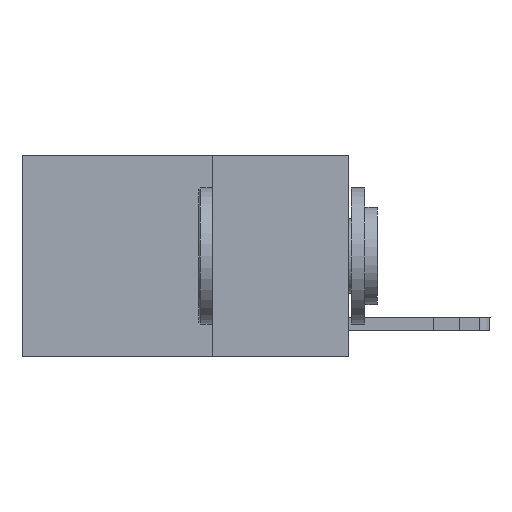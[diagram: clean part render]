
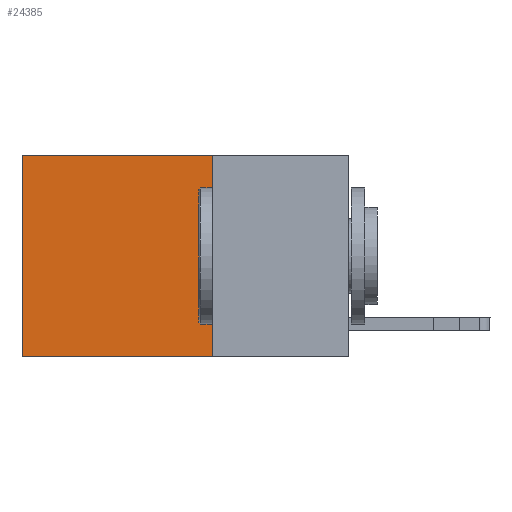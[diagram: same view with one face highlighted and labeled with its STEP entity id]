
A CAD part, left-side view. The second image highlights one B-rep face of the part: STEP entity #24385.
In plain terms, the highlighted planar face has unit normal (-1, 0, 0).
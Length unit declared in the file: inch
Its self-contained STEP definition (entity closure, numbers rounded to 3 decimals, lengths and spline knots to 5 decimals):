
#61 = ORIENTED_EDGE ( 'NONE', *, *, #6524, .T. ) ;
#333 = FACE_OUTER_BOUND ( 'NONE', #22624, .T. ) ;
#690 = EDGE_CURVE ( 'NONE', #24921, #1788, #8399, .T. ) ;
#1788 = VERTEX_POINT ( 'NONE', #17056 ) ;
#2636 = AXIS2_PLACEMENT_3D ( 'NONE', #22788, #10754, #24812 ) ;
#2670 = EDGE_CURVE ( 'NONE', #4900, #24490, #13445, .T. ) ;
#2940 = CARTESIAN_POINT ( 'NONE',  ( 0.2625, 0.6, 0. ) ) ;
#4840 = DIRECTION ( 'NONE',  ( 0., 0., -1. ) ) ;
#4900 = VERTEX_POINT ( 'NONE', #12965 ) ;
#5630 = CARTESIAN_POINT ( 'NONE',  ( 0.2625, 0.25, 0. ) ) ;
#6524 = EDGE_CURVE ( 'NONE', #24490, #1788, #13587, .T. ) ;
#7701 = DIRECTION ( 'NONE',  ( 0., 1., 0. ) ) ;
#7857 = CARTESIAN_POINT ( 'NONE',  ( 0.2625, 0.25, 0. ) ) ;
#8399 = LINE ( 'NONE', #25660, #13099 ) ;
#10754 = DIRECTION ( 'NONE',  ( 1., 0., 0. ) ) ;
#11205 = VECTOR ( 'NONE', #15688, 39.37008 ) ;
#12495 = EDGE_CURVE ( 'NONE', #4900, #24921, #21913, .T. ) ;
#12965 = CARTESIAN_POINT ( 'NONE',  ( 0.2625, 0.25, 0. ) ) ;
#13099 = VECTOR ( 'NONE', #25542, 39.37008 ) ;
#13445 = LINE ( 'NONE', #7857, #18806 ) ;
#13587 = LINE ( 'NONE', #16914, #24276 ) ;
#14439 = CARTESIAN_POINT ( 'NONE',  ( 0.2625, 0.25, -0.37 ) ) ;
#15688 = DIRECTION ( 'NONE',  ( 0., 0., -1. ) ) ;
#16728 = PLANE ( 'NONE',  #2636 ) ;
#16914 = CARTESIAN_POINT ( 'NONE',  ( 0.2625, 0.6, 0. ) ) ;
#17056 = CARTESIAN_POINT ( 'NONE',  ( 0.2625, 0.6, -0.37 ) ) ;
#18497 = ORIENTED_EDGE ( 'NONE', *, *, #2670, .T. ) ;
#18806 = VECTOR ( 'NONE', #7701, 39.37008 ) ;
#20195 = ORIENTED_EDGE ( 'NONE', *, *, #12495, .F. ) ;
#21028 = ORIENTED_EDGE ( 'NONE', *, *, #690, .F. ) ;
#21913 = LINE ( 'NONE', #5630, #11205 ) ;
#22624 = EDGE_LOOP ( 'NONE', ( #61, #21028, #20195, #18497 ) ) ;
#22788 = CARTESIAN_POINT ( 'NONE',  ( 0.2625, 0.25, 0. ) ) ;
#24276 = VECTOR ( 'NONE', #4840, 39.37008 ) ;
#24385 = ADVANCED_FACE ( 'NONE', ( #333 ), #16728, .F. ) ;
#24490 = VERTEX_POINT ( 'NONE', #2940 ) ;
#24812 = DIRECTION ( 'NONE',  ( 0., 0., -1. ) ) ;
#24921 = VERTEX_POINT ( 'NONE', #14439 ) ;
#25542 = DIRECTION ( 'NONE',  ( 0., 1., 0. ) ) ;
#25660 = CARTESIAN_POINT ( 'NONE',  ( 0.2625, 0.25, -0.37 ) ) ;
